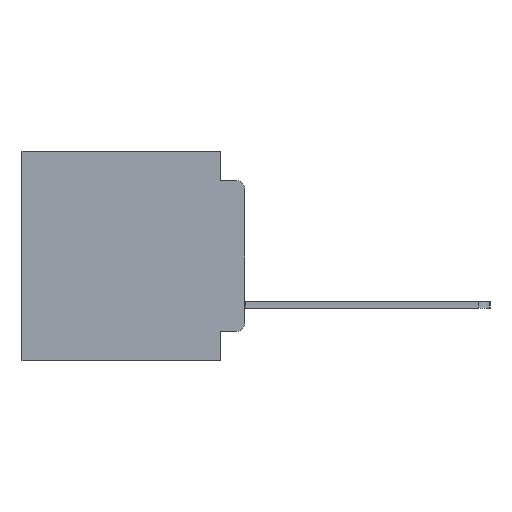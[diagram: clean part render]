
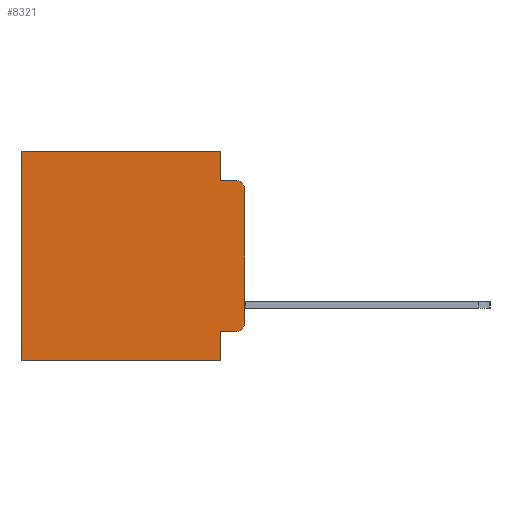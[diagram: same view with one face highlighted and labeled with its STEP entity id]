
A CAD part, left-side view. The second image highlights one B-rep face of the part: STEP entity #8321.
In plain terms, the highlighted planar face has unit normal (-1, 0, 0).
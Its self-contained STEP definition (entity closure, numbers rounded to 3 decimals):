
#258 = VECTOR ( 'NONE', #5421, 1000. ) ;
#760 = EDGE_CURVE ( 'NONE', #20776, #18632, #10330, .T. ) ;
#1866 = DIRECTION ( 'NONE',  ( 0., -1., 0. ) ) ;
#2288 = CARTESIAN_POINT ( 'NONE',  ( -67.462, 1.295, 0. ) ) ;
#2387 = DIRECTION ( 'NONE',  ( 0., 0., -1. ) ) ;
#2418 = ORIENTED_EDGE ( 'NONE', *, *, #760, .F. ) ;
#3706 = ORIENTED_EDGE ( 'NONE', *, *, #15182, .T. ) ;
#3896 = EDGE_CURVE ( 'NONE', #10100, #5914, #7357, .T. ) ;
#4592 = CARTESIAN_POINT ( 'NONE',  ( -67.462, 1.295, -5.486 ) ) ;
#4695 = AXIS2_PLACEMENT_3D ( 'NONE', #11180, #24255, #26047 ) ;
#5212 = CARTESIAN_POINT ( 'NONE',  ( -67.462, 11.684, -5.486 ) ) ;
#5353 = VECTOR ( 'NONE', #19605, 1000. ) ;
#5421 = DIRECTION ( 'NONE',  ( 0., 1., 0. ) ) ;
#5818 = ORIENTED_EDGE ( 'NONE', *, *, #23954, .F. ) ;
#5914 = VERTEX_POINT ( 'NONE', #22785 ) ;
#6135 = CARTESIAN_POINT ( 'NONE',  ( -67.462, 0.508, -3.467 ) ) ;
#6252 = VECTOR ( 'NONE', #14011, 1000. ) ;
#6277 = ORIENTED_EDGE ( 'NONE', *, *, #8853, .T. ) ;
#7357 = LINE ( 'NONE', #24733, #258 ) ;
#7862 = VERTEX_POINT ( 'NONE', #27593 ) ;
#8256 = VECTOR ( 'NONE', #15266, 1000. ) ;
#8321 = ADVANCED_FACE ( 'NONE', ( #17326 ), #11094, .F. ) ;
#8519 = EDGE_LOOP ( 'NONE', ( #6277, #3706, #2418, #19978, #5818, #18453, #12177, #17871, #16998, #12420 ) ) ;
#8607 = DIRECTION ( 'NONE',  ( 0., 0., -1. ) ) ;
#8853 = EDGE_CURVE ( 'NONE', #7862, #19225, #9372, .T. ) ;
#9372 = LINE ( 'NONE', #10786, #5353 ) ;
#10100 = VERTEX_POINT ( 'NONE', #4592 ) ;
#10330 = LINE ( 'NONE', #15257, #14753 ) ;
#10673 = LINE ( 'NONE', #5212, #6252 ) ;
#10786 = CARTESIAN_POINT ( 'NONE',  ( -67.462, 1.295, -3.975 ) ) ;
#10818 = LINE ( 'NONE', #16856, #20981 ) ;
#11094 = PLANE ( 'NONE',  #4695 ) ;
#11180 = CARTESIAN_POINT ( 'NONE',  ( -67.462, 0., -5.486 ) ) ;
#12177 = ORIENTED_EDGE ( 'NONE', *, *, #26593, .T. ) ;
#12420 = ORIENTED_EDGE ( 'NONE', *, *, #22713, .F. ) ;
#13080 = CARTESIAN_POINT ( 'NONE',  ( -67.462, 0., 5.486 ) ) ;
#14011 = DIRECTION ( 'NONE',  ( 0., 0., -1. ) ) ;
#14753 = VECTOR ( 'NONE', #8607, 1000. ) ;
#14894 = EDGE_CURVE ( 'NONE', #22989, #5914, #10673, .T. ) ;
#15182 = EDGE_CURVE ( 'NONE', #19225, #18632, #15509, .T. ) ;
#15257 = CARTESIAN_POINT ( 'NONE',  ( -67.462, 0., -5.486 ) ) ;
#15266 = DIRECTION ( 'NONE',  ( 0., 1., 0. ) ) ;
#15509 = CIRCLE ( 'NONE', #23835, 0.508 ) ;
#15559 = CARTESIAN_POINT ( 'NONE',  ( -67.462, 1.295, 0. ) ) ;
#16461 = CARTESIAN_POINT ( 'NONE',  ( -67.462, 0.508, 3.467 ) ) ;
#16659 = CARTESIAN_POINT ( 'NONE',  ( -67.462, 0., -3.467 ) ) ;
#16856 = CARTESIAN_POINT ( 'NONE',  ( -67.462, 1.295, 3.975 ) ) ;
#16932 = CARTESIAN_POINT ( 'NONE',  ( -67.462, 0., 3.467 ) ) ;
#16998 = ORIENTED_EDGE ( 'NONE', *, *, #3896, .F. ) ;
#17186 = CARTESIAN_POINT ( 'NONE',  ( -67.462, 1.295, 5.486 ) ) ;
#17221 = DIRECTION ( 'NONE',  ( 0., 0., -1. ) ) ;
#17326 = FACE_OUTER_BOUND ( 'NONE', #8519, .T. ) ;
#17577 = AXIS2_PLACEMENT_3D ( 'NONE', #16461, #20892, #24781 ) ;
#17643 = LINE ( 'NONE', #2288, #17990 ) ;
#17871 = ORIENTED_EDGE ( 'NONE', *, *, #14894, .T. ) ;
#17990 = VECTOR ( 'NONE', #2387, 1000. ) ;
#18453 = ORIENTED_EDGE ( 'NONE', *, *, #19295, .F. ) ;
#18632 = VERTEX_POINT ( 'NONE', #16659 ) ;
#19225 = VERTEX_POINT ( 'NONE', #21046 ) ;
#19295 = EDGE_CURVE ( 'NONE', #21418, #19725, #17643, .T. ) ;
#19305 = DIRECTION ( 'NONE',  ( -1., 0., 0. ) ) ;
#19461 = CARTESIAN_POINT ( 'NONE',  ( -67.462, 11.684, 5.486 ) ) ;
#19605 = DIRECTION ( 'NONE',  ( 0., -1., 0. ) ) ;
#19725 = VERTEX_POINT ( 'NONE', #27980 ) ;
#19978 = ORIENTED_EDGE ( 'NONE', *, *, #20645, .T. ) ;
#20391 = VECTOR ( 'NONE', #26782, 1000. ) ;
#20645 = EDGE_CURVE ( 'NONE', #20776, #27586, #26687, .T. ) ;
#20776 = VERTEX_POINT ( 'NONE', #16932 ) ;
#20892 = DIRECTION ( 'NONE',  ( -1., 0., 0. ) ) ;
#20981 = VECTOR ( 'NONE', #1866, 1000. ) ;
#21046 = CARTESIAN_POINT ( 'NONE',  ( -67.462, 0.508, -3.975 ) ) ;
#21418 = VERTEX_POINT ( 'NONE', #17186 ) ;
#21735 = LINE ( 'NONE', #15559, #20391 ) ;
#22713 = EDGE_CURVE ( 'NONE', #7862, #10100, #21735, .T. ) ;
#22785 = CARTESIAN_POINT ( 'NONE',  ( -67.462, 11.684, -5.486 ) ) ;
#22989 = VERTEX_POINT ( 'NONE', #19461 ) ;
#23835 = AXIS2_PLACEMENT_3D ( 'NONE', #6135, #19305, #17221 ) ;
#23954 = EDGE_CURVE ( 'NONE', #19725, #27586, #10818, .T. ) ;
#24255 = DIRECTION ( 'NONE',  ( 1., 0., 0. ) ) ;
#24733 = CARTESIAN_POINT ( 'NONE',  ( -67.462, 0., -5.486 ) ) ;
#24781 = DIRECTION ( 'NONE',  ( 0., 0., -1. ) ) ;
#25535 = LINE ( 'NONE', #13080, #8256 ) ;
#26047 = DIRECTION ( 'NONE',  ( 0., 0., -1. ) ) ;
#26593 = EDGE_CURVE ( 'NONE', #21418, #22989, #25535, .T. ) ;
#26687 = CIRCLE ( 'NONE', #17577, 0.508 ) ;
#26782 = DIRECTION ( 'NONE',  ( 0., 0., -1. ) ) ;
#27120 = CARTESIAN_POINT ( 'NONE',  ( -67.462, 0.508, 3.975 ) ) ;
#27586 = VERTEX_POINT ( 'NONE', #27120 ) ;
#27593 = CARTESIAN_POINT ( 'NONE',  ( -67.462, 1.295, -3.975 ) ) ;
#27980 = CARTESIAN_POINT ( 'NONE',  ( -67.462, 1.295, 3.975 ) ) ;
